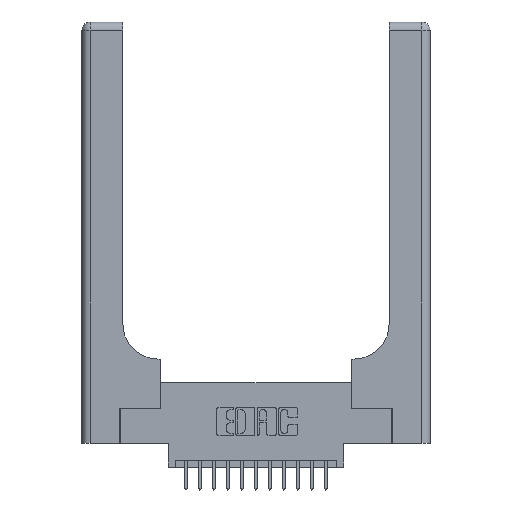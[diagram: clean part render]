
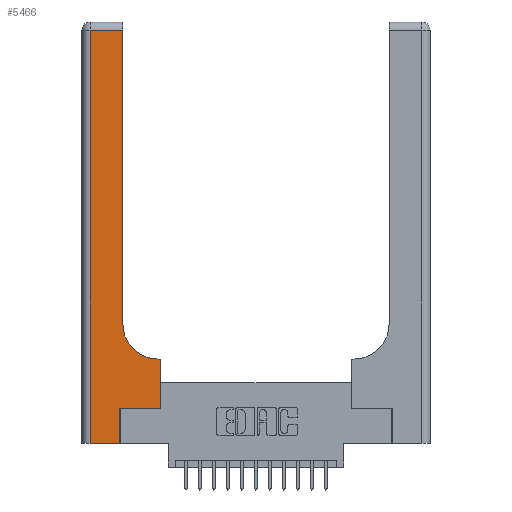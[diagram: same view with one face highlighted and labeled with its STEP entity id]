
A CAD part, top view. The second image highlights one B-rep face of the part: STEP entity #5466.
In plain terms, the highlighted planar face has unit normal (0, 0, 1).
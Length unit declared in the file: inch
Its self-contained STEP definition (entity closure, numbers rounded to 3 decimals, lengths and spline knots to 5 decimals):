
#50 = ORIENTED_EDGE ( 'NONE', *, *, #4737, .T. ) ;
#171 = CARTESIAN_POINT ( 'NONE',  ( 0.2915, 0.6, 0.37 ) ) ;
#331 = CARTESIAN_POINT ( 'NONE',  ( 0.269, 0.25, 0.37 ) ) ;
#371 = ORIENTED_EDGE ( 'NONE', *, *, #4259, .T. ) ;
#678 = VECTOR ( 'NONE', #17019, 39.37008 ) ;
#997 = FACE_OUTER_BOUND ( 'NONE', #11169, .T. ) ;
#1031 = VECTOR ( 'NONE', #16051, 39.37008 ) ;
#1090 = CARTESIAN_POINT ( 'NONE',  ( 0., 3., 0.37 ) ) ;
#1167 = VERTEX_POINT ( 'NONE', #9211 ) ;
#1757 = LINE ( 'NONE', #331, #15803 ) ;
#1786 = LINE ( 'NONE', #12280, #16257 ) ;
#1857 = AXIS2_PLACEMENT_3D ( 'NONE', #11466, #3138, #12884 ) ;
#1918 = ORIENTED_EDGE ( 'NONE', *, *, #3753, .T. ) ;
#2043 = VERTEX_POINT ( 'NONE', #17621 ) ;
#2267 = CARTESIAN_POINT ( 'NONE',  ( 0.269, 0., 0.37 ) ) ;
#2552 = VERTEX_POINT ( 'NONE', #4522 ) ;
#2561 = DIRECTION ( 'NONE',  ( -1., 0., 0. ) ) ;
#2764 = ORIENTED_EDGE ( 'NONE', *, *, #14608, .T. ) ;
#3138 = DIRECTION ( 'NONE',  ( 0., 0., -1. ) ) ;
#3745 = LINE ( 'NONE', #12875, #10666 ) ;
#3753 = EDGE_CURVE ( 'NONE', #2552, #12027, #1757, .T. ) ;
#3973 = DIRECTION ( 'NONE',  ( 0., 1., 0. ) ) ;
#4068 = LINE ( 'NONE', #2267, #14748 ) ;
#4259 = EDGE_CURVE ( 'NONE', #16996, #9291, #15787, .T. ) ;
#4311 = AXIS2_PLACEMENT_3D ( 'NONE', #1090, #10909, #2561 ) ;
#4522 = CARTESIAN_POINT ( 'NONE',  ( 0.269, 0.25, 0.37 ) ) ;
#4737 = EDGE_CURVE ( 'NONE', #12027, #1167, #5119, .T. ) ;
#4959 = CARTESIAN_POINT ( 'NONE',  ( 0.2915, 0.85, 0.37 ) ) ;
#5119 = LINE ( 'NONE', #15186, #12020 ) ;
#5169 = CARTESIAN_POINT ( 'NONE',  ( 0.2915, 2.94, 0.37 ) ) ;
#5466 = ADVANCED_FACE ( 'NONE', ( #997 ), #6748, .F. ) ;
#6003 = ORIENTED_EDGE ( 'NONE', *, *, #10673, .T. ) ;
#6286 = ORIENTED_EDGE ( 'NONE', *, *, #9857, .T. ) ;
#6479 = DIRECTION ( 'NONE',  ( 0., 1., 0. ) ) ;
#6529 = VECTOR ( 'NONE', #16999, 39.37008 ) ;
#6748 = PLANE ( 'NONE',  #4311 ) ;
#6967 = VERTEX_POINT ( 'NONE', #5169 ) ;
#7679 = CARTESIAN_POINT ( 'NONE',  ( 0., 0., 0.37 ) ) ;
#8189 = LINE ( 'NONE', #171, #678 ) ;
#8221 = DIRECTION ( 'NONE',  ( 0., 1., 0. ) ) ;
#8227 = EDGE_CURVE ( 'NONE', #9291, #6967, #1786, .T. ) ;
#8965 = VERTEX_POINT ( 'NONE', #15340 ) ;
#9211 = CARTESIAN_POINT ( 'NONE',  ( 0.5585, 0.6, 0.37 ) ) ;
#9291 = VERTEX_POINT ( 'NONE', #4959 ) ;
#9649 = ORIENTED_EDGE ( 'NONE', *, *, #8227, .T. ) ;
#9857 = EDGE_CURVE ( 'NONE', #8965, #2043, #12236, .T. ) ;
#10666 = VECTOR ( 'NONE', #14285, 39.37008 ) ;
#10673 = EDGE_CURVE ( 'NONE', #6967, #17548, #3745, .T. ) ;
#10773 = ORIENTED_EDGE ( 'NONE', *, *, #17246, .T. ) ;
#10909 = DIRECTION ( 'NONE',  ( 0., 0., -1. ) ) ;
#11169 = EDGE_LOOP ( 'NONE', ( #9649, #6003, #2764, #6286, #10773, #1918, #50, #11263, #371 ) ) ;
#11263 = ORIENTED_EDGE ( 'NONE', *, *, #15990, .T. ) ;
#11412 = CARTESIAN_POINT ( 'NONE',  ( 0.5585, 0.25, 0.37 ) ) ;
#11466 = CARTESIAN_POINT ( 'NONE',  ( 0.5415, 0.85, 0.37 ) ) ;
#12020 = VECTOR ( 'NONE', #8221, 39.37008 ) ;
#12027 = VERTEX_POINT ( 'NONE', #11412 ) ;
#12236 = LINE ( 'NONE', #7679, #1031 ) ;
#12280 = CARTESIAN_POINT ( 'NONE',  ( 0.2915, 3., 0.37 ) ) ;
#12875 = CARTESIAN_POINT ( 'NONE',  ( 0., 2.94, 0.37 ) ) ;
#12884 = DIRECTION ( 'NONE',  ( 1., 0., 0. ) ) ;
#14283 = CARTESIAN_POINT ( 'NONE',  ( 0.5415, 0.6, 0.37 ) ) ;
#14285 = DIRECTION ( 'NONE',  ( -1., 0., 0. ) ) ;
#14608 = EDGE_CURVE ( 'NONE', #17548, #8965, #17633, .T. ) ;
#14748 = VECTOR ( 'NONE', #6479, 39.37008 ) ;
#15186 = CARTESIAN_POINT ( 'NONE',  ( 0.5585, 0.25, 0.37 ) ) ;
#15340 = CARTESIAN_POINT ( 'NONE',  ( 0.06, 0., 0.37 ) ) ;
#15368 = CARTESIAN_POINT ( 'NONE',  ( 0.06, 2.94, 0.37 ) ) ;
#15612 = CARTESIAN_POINT ( 'NONE',  ( 0.06, 3., 0.37 ) ) ;
#15787 = CIRCLE ( 'NONE', #1857, 0.25 ) ;
#15803 = VECTOR ( 'NONE', #15854, 39.37008 ) ;
#15854 = DIRECTION ( 'NONE',  ( 1., 0., 0. ) ) ;
#15990 = EDGE_CURVE ( 'NONE', #1167, #16996, #8189, .T. ) ;
#16051 = DIRECTION ( 'NONE',  ( 1., 0., 0. ) ) ;
#16257 = VECTOR ( 'NONE', #3973, 39.37008 ) ;
#16996 = VERTEX_POINT ( 'NONE', #14283 ) ;
#16999 = DIRECTION ( 'NONE',  ( 0., -1., 0. ) ) ;
#17019 = DIRECTION ( 'NONE',  ( -1., 0., 0. ) ) ;
#17246 = EDGE_CURVE ( 'NONE', #2043, #2552, #4068, .T. ) ;
#17548 = VERTEX_POINT ( 'NONE', #15368 ) ;
#17621 = CARTESIAN_POINT ( 'NONE',  ( 0.269, 0., 0.37 ) ) ;
#17633 = LINE ( 'NONE', #15612, #6529 ) ;
